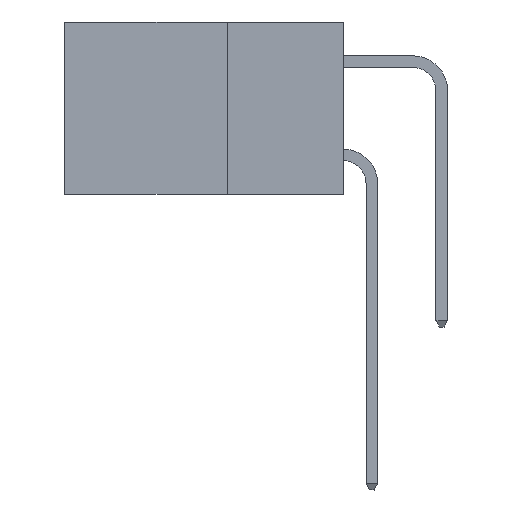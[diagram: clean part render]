
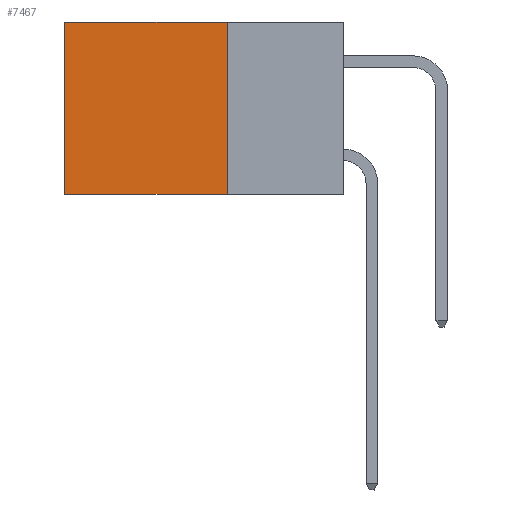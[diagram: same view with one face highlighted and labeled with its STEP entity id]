
A CAD part, left-side view. The second image highlights one B-rep face of the part: STEP entity #7467.
In plain terms, the highlighted planar face has unit normal (-1, 0, 0).
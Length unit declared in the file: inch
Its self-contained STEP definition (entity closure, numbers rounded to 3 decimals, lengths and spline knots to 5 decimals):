
#707 = ORIENTED_EDGE ( 'NONE', *, *, #11693, .T. ) ;
#708 = EDGE_CURVE ( 'NONE', #10695, #13035, #6234, .T. ) ;
#1585 = ORIENTED_EDGE ( 'NONE', *, *, #708, .F. ) ;
#4953 = EDGE_CURVE ( 'NONE', #16083, #12509, #9313, .T. ) ;
#4969 = CARTESIAN_POINT ( 'NONE',  ( 0.298, 0.25, 0. ) ) ;
#5909 = VECTOR ( 'NONE', #9287, 39.37008 ) ;
#5947 = DIRECTION ( 'NONE',  ( 0., 0., -1. ) ) ;
#5969 = DIRECTION ( 'NONE',  ( 1., 0., 0. ) ) ;
#6006 = CARTESIAN_POINT ( 'NONE',  ( 0.298, 0.25, 0. ) ) ;
#6032 = PLANE ( 'NONE',  #6778 ) ;
#6234 = LINE ( 'NONE', #8911, #16038 ) ;
#6778 = AXIS2_PLACEMENT_3D ( 'NONE', #6006, #5969, #5947 ) ;
#7467 = ADVANCED_FACE ( 'NONE', ( #8038 ), #6032, .F. ) ;
#7991 = CARTESIAN_POINT ( 'NONE',  ( 0.298, 0.25, 0. ) ) ;
#8038 = FACE_OUTER_BOUND ( 'NONE', #14496, .T. ) ;
#8112 = CARTESIAN_POINT ( 'NONE',  ( 0.298, 0.25, -0.37 ) ) ;
#8907 = DIRECTION ( 'NONE',  ( 0., 1., 0. ) ) ;
#8911 = CARTESIAN_POINT ( 'NONE',  ( 0.298, 0.25, -0.37 ) ) ;
#9287 = DIRECTION ( 'NONE',  ( 0., 0., -1. ) ) ;
#9313 = LINE ( 'NONE', #16714, #15323 ) ;
#10092 = DIRECTION ( 'NONE',  ( 0., 1., 0. ) ) ;
#10495 = ORIENTED_EDGE ( 'NONE', *, *, #4953, .T. ) ;
#10543 = VECTOR ( 'NONE', #16682, 39.37008 ) ;
#10688 = CARTESIAN_POINT ( 'NONE',  ( 0.298, 0.6, 0. ) ) ;
#10695 = VERTEX_POINT ( 'NONE', #8112 ) ;
#10974 = ORIENTED_EDGE ( 'NONE', *, *, #16765, .F. ) ;
#11693 = EDGE_CURVE ( 'NONE', #12509, #13035, #13955, .T. ) ;
#12509 = VERTEX_POINT ( 'NONE', #10688 ) ;
#13035 = VERTEX_POINT ( 'NONE', #14327 ) ;
#13955 = LINE ( 'NONE', #15369, #10543 ) ;
#14327 = CARTESIAN_POINT ( 'NONE',  ( 0.298, 0.6, -0.37 ) ) ;
#14496 = EDGE_LOOP ( 'NONE', ( #707, #1585, #10974, #10495 ) ) ;
#15323 = VECTOR ( 'NONE', #10092, 39.37008 ) ;
#15369 = CARTESIAN_POINT ( 'NONE',  ( 0.298, 0.6, 0. ) ) ;
#16038 = VECTOR ( 'NONE', #8907, 39.37008 ) ;
#16083 = VERTEX_POINT ( 'NONE', #4969 ) ;
#16124 = LINE ( 'NONE', #7991, #5909 ) ;
#16682 = DIRECTION ( 'NONE',  ( 0., 0., -1. ) ) ;
#16714 = CARTESIAN_POINT ( 'NONE',  ( 0.298, 0.25, 0. ) ) ;
#16765 = EDGE_CURVE ( 'NONE', #16083, #10695, #16124, .T. ) ;
